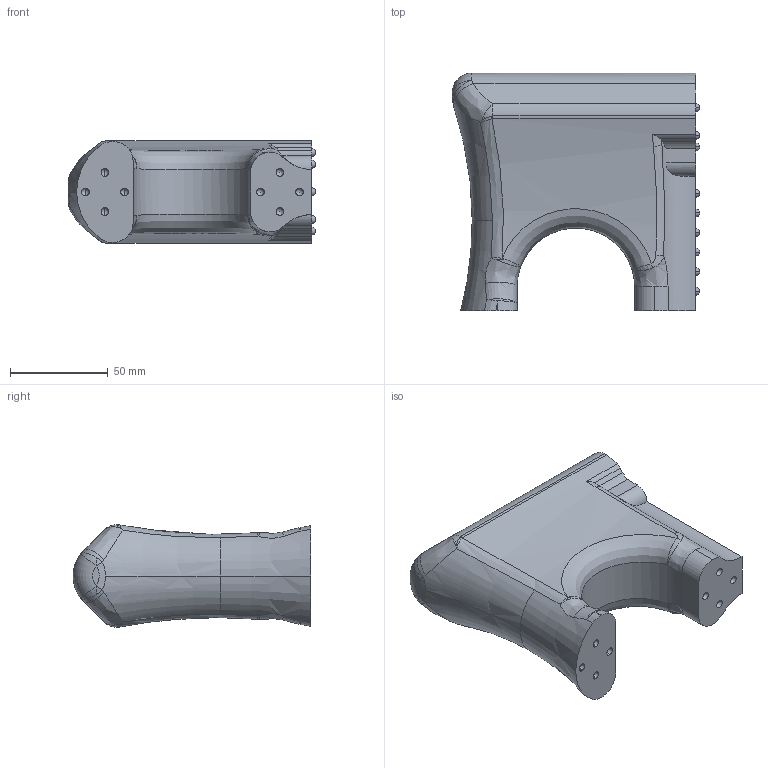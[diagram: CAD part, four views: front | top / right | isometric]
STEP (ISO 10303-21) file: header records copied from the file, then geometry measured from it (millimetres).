
FILE_DESCRIPTION (( 'STEP AP214' ), '1' );
FILE_NAME ('Stock Rear.STEP', '2013-06-24T22:47:41', ( 'Asher' ), ( '' ), 'SwSTEP 2.0', 'SolidWorks 2013', '' );
FILE_SCHEMA (( 'AUTOMOTIVE_DESIGN' ));
Length unit declared in the file: millimetre
Products named in the file (1): Stock Rear
Bounding box: 126.3 x 121.45 x 52.5 mm (x, y, z)
Volume: 439442.6 mm3; surface area: 47993.7 mm2
Topology: 1 solids, 1 shells, 127 faces, 356 edges, 213 vertices
Faces by surface type: sphere 48, bspline 31, cylinder 28, plane 13, torus 7
Entity records: 6120 total; most frequent: CARTESIAN_POINT 3462, ORIENTED_EDGE 560, DIRECTION 525, EDGE_CURVE 280, AXIS2_PLACEMENT_3D 239, VERTEX_POINT 175, EDGE_LOOP 147, CIRCLE 142
